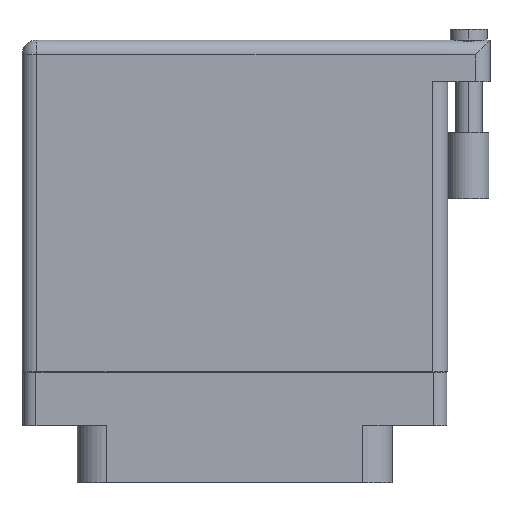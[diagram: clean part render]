
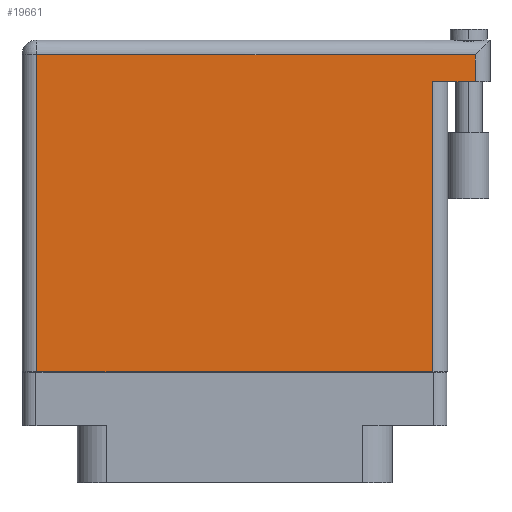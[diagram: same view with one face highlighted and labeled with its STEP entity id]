
A CAD part, front view. The second image highlights one B-rep face of the part: STEP entity #19661.
In plain terms, the highlighted face is planar.
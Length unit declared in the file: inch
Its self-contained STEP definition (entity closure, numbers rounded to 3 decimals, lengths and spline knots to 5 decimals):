
#141 = VECTOR ( 'NONE', #15612, 39.37008 ) ;
#356 = ORIENTED_EDGE ( 'NONE', *, *, #31817, .T. ) ;
#1148 = CARTESIAN_POINT ( 'NONE',  ( -1.004, 1.396, 0.4495 ) ) ;
#1649 = EDGE_CURVE ( 'NONE', #15982, #16030, #32437, .T. ) ;
#1846 = VECTOR ( 'NONE', #22031, 39.37008 ) ;
#1898 = CARTESIAN_POINT ( 'NONE',  ( 1.134, 1.466, 0.4495 ) ) ;
#2560 = PLANE ( 'NONE',  #10233 ) ;
#2807 = DIRECTION ( 'NONE',  ( 0., 0., -1. ) ) ;
#3006 = DIRECTION ( 'NONE',  ( -1., 0., 0. ) ) ;
#3984 = VERTEX_POINT ( 'NONE', #32134 ) ;
#5568 = CARTESIAN_POINT ( 'NONE',  ( -0.934, -0.1, 0.4495 ) ) ;
#5601 = DIRECTION ( 'NONE',  ( -1., 0., 0. ) ) ;
#7142 = CARTESIAN_POINT ( 'NONE',  ( -1.004, 1.466, 0.4495 ) ) ;
#7311 = CARTESIAN_POINT ( 'NONE',  ( -0.934, -0.1, 0.4495 ) ) ;
#7450 = FACE_OUTER_BOUND ( 'NONE', #10187, .T. ) ;
#7842 = DIRECTION ( 'NONE',  ( 0., 1., 0. ) ) ;
#7953 = CARTESIAN_POINT ( 'NONE',  ( -0.934, 1.396, 0.4495 ) ) ;
#8083 = LINE ( 'NONE', #1898, #35642 ) ;
#8325 = ORIENTED_EDGE ( 'NONE', *, *, #17790, .T. ) ;
#8955 = ORIENTED_EDGE ( 'NONE', *, *, #16576, .T. ) ;
#9637 = LINE ( 'NONE', #7311, #141 ) ;
#9956 = VECTOR ( 'NONE', #12111, 39.37008 ) ;
#10187 = EDGE_LOOP ( 'NONE', ( #16371, #28141, #15919, #8955, #8325, #356 ) ) ;
#10233 = AXIS2_PLACEMENT_3D ( 'NONE', #7142, #2807, #5601 ) ;
#11023 = CARTESIAN_POINT ( 'NONE',  ( 0.934, 1.269, 0.4495 ) ) ;
#11674 = CARTESIAN_POINT ( 'NONE',  ( 0.934, -0.1, 0.4495 ) ) ;
#12111 = DIRECTION ( 'NONE',  ( 1., 0., 0. ) ) ;
#13804 = CARTESIAN_POINT ( 'NONE',  ( 1.204, 1.269, 0.4495 ) ) ;
#15612 = DIRECTION ( 'NONE',  ( 0., -1., 0. ) ) ;
#15919 = ORIENTED_EDGE ( 'NONE', *, *, #20892, .F. ) ;
#15982 = VERTEX_POINT ( 'NONE', #5568 ) ;
#16030 = VERTEX_POINT ( 'NONE', #11674 ) ;
#16371 = ORIENTED_EDGE ( 'NONE', *, *, #1649, .T. ) ;
#16576 = EDGE_CURVE ( 'NONE', #3984, #34680, #8083, .T. ) ;
#17790 = EDGE_CURVE ( 'NONE', #34680, #18678, #19606, .T. ) ;
#17813 = LINE ( 'NONE', #33392, #1846 ) ;
#18079 = VECTOR ( 'NONE', #3006, 39.37008 ) ;
#18678 = VERTEX_POINT ( 'NONE', #7953 ) ;
#18728 = VECTOR ( 'NONE', #20459, 39.37008 ) ;
#19374 = LINE ( 'NONE', #13804, #18079 ) ;
#19606 = LINE ( 'NONE', #1148, #18728 ) ;
#19661 = ADVANCED_FACE ( 'NONE', ( #7450 ), #2560, .F. ) ;
#20459 = DIRECTION ( 'NONE',  ( -1., 0., 0. ) ) ;
#20892 = EDGE_CURVE ( 'NONE', #3984, #34579, #19374, .T. ) ;
#22031 = DIRECTION ( 'NONE',  ( 0., 1., 0. ) ) ;
#26020 = CARTESIAN_POINT ( 'NONE',  ( -1.004, -0.1, 0.4495 ) ) ;
#28141 = ORIENTED_EDGE ( 'NONE', *, *, #31562, .T. ) ;
#31562 = EDGE_CURVE ( 'NONE', #16030, #34579, #17813, .T. ) ;
#31817 = EDGE_CURVE ( 'NONE', #18678, #15982, #9637, .T. ) ;
#32134 = CARTESIAN_POINT ( 'NONE',  ( 1.134, 1.269, 0.4495 ) ) ;
#32437 = LINE ( 'NONE', #26020, #9956 ) ;
#33228 = CARTESIAN_POINT ( 'NONE',  ( 1.134, 1.396, 0.4495 ) ) ;
#33392 = CARTESIAN_POINT ( 'NONE',  ( 0.934, 1.269, 0.4495 ) ) ;
#34579 = VERTEX_POINT ( 'NONE', #11023 ) ;
#34680 = VERTEX_POINT ( 'NONE', #33228 ) ;
#35642 = VECTOR ( 'NONE', #7842, 39.37008 ) ;
